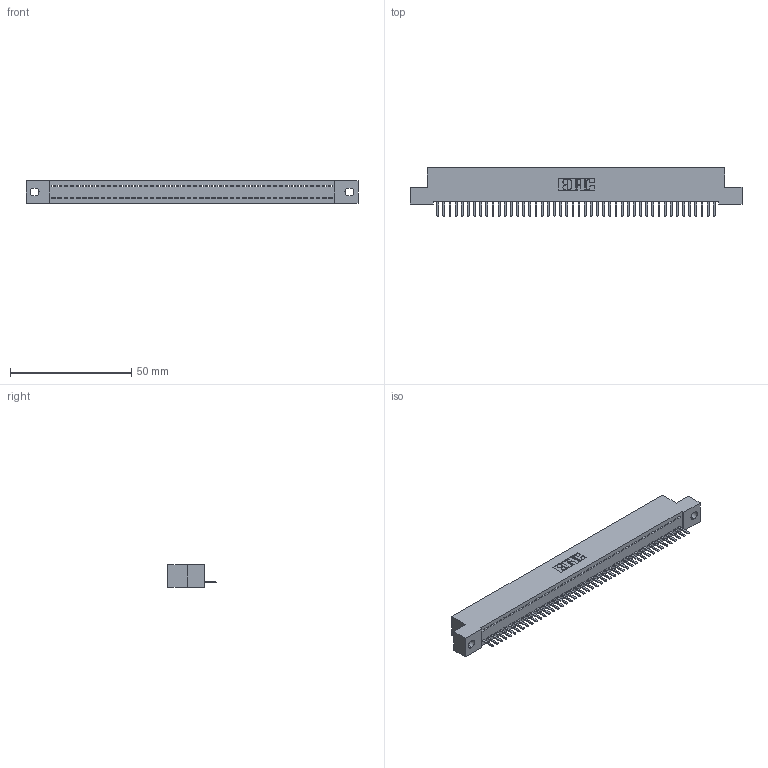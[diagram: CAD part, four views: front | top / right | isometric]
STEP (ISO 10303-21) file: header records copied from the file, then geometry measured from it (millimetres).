
FILE_DESCRIPTION (( 'STEP AP203' ), '1' );
FILE_NAME ('342-046-520-102.STEP', '2019-10-02T20:12:24', ( '' ), ( '' ), 'SwSTEP 2.0', 'SolidWorks 2016', '' );
FILE_SCHEMA (( 'CONFIG_CONTROL_DESIGN' ));
Length unit declared in the file: inch
Products named in the file (3): 342 Part_.128 Slot; 345-292-001_345-293-120; 342-046-520-102
Assembly tree (47 placements, depth 2):
  342-046-520-102
    342 Part_.128 Slot
    345-292-001_345-293-120  x46
Bounding box: 137.16 x 20.02 x 9.4 mm (x, y, z)
Volume: 11856.5 mm3; surface area: 16821.8 mm2
Topology: 47 solids, 47 shells, 2966 faces, 8775 edges, 5726 vertices
Faces by surface type: plane 2094, cylinder 872
Entity records: 27721 total; most frequent: CARTESIAN_POINT 4800, ORIENTED_EDGE 4770, DIRECTION 4029, EDGE_CURVE 2385, VECTOR 2253, LINE 2253, VERTEX_POINT 1586, AXIS2_PLACEMENT_3D 888
